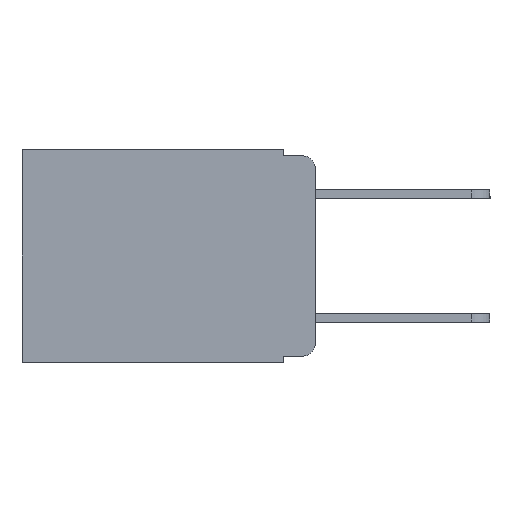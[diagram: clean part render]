
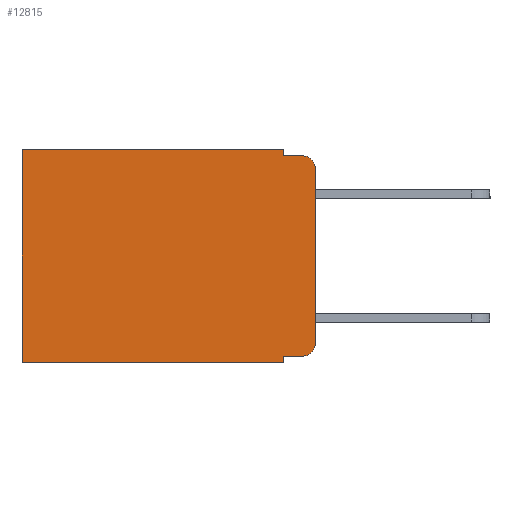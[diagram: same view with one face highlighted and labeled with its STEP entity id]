
A CAD part, left-side view. The second image highlights one B-rep face of the part: STEP entity #12815.
In plain terms, the highlighted planar face has unit normal (-1, 0, 0).
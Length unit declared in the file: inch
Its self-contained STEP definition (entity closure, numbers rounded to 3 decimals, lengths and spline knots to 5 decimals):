
#203 = LINE ( 'NONE', #10145, #24065 ) ;
#232 = AXIS2_PLACEMENT_3D ( 'NONE', #9167, #1278, #14845 ) ;
#376 = FACE_OUTER_BOUND ( 'NONE', #3864, .T. ) ;
#669 = CARTESIAN_POINT ( 'NONE',  ( 0.298, 0.02, -0.01 ) ) ;
#737 = DIRECTION ( 'NONE',  ( 0., 0., -1. ) ) ;
#932 = EDGE_CURVE ( 'NONE', #7446, #4403, #10156, .T. ) ;
#989 = CARTESIAN_POINT ( 'NONE',  ( 0.298, 0.051, -0.333 ) ) ;
#1278 = DIRECTION ( 'NONE',  ( 1., 0., 0. ) ) ;
#1510 = VERTEX_POINT ( 'NONE', #11064 ) ;
#1795 = CARTESIAN_POINT ( 'NONE',  ( 0.298, 0.051, 0. ) ) ;
#1995 = CARTESIAN_POINT ( 'NONE',  ( 0.298, 0.051, -0.01 ) ) ;
#2602 = ORIENTED_EDGE ( 'NONE', *, *, #932, .F. ) ;
#2742 = DIRECTION ( 'NONE',  ( 0., 1., 0. ) ) ;
#3215 = VERTEX_POINT ( 'NONE', #3686 ) ;
#3256 = ORIENTED_EDGE ( 'NONE', *, *, #9403, .T. ) ;
#3280 = ORIENTED_EDGE ( 'NONE', *, *, #9999, .F. ) ;
#3568 = ORIENTED_EDGE ( 'NONE', *, *, #19341, .F. ) ;
#3686 = CARTESIAN_POINT ( 'NONE',  ( 0.298, 0.473, 0. ) ) ;
#3766 = LINE ( 'NONE', #22955, #8368 ) ;
#3864 = EDGE_LOOP ( 'NONE', ( #22841, #7643, #3568, #2602, #13840, #3256, #3280, #7312, #7011, #20078 ) ) ;
#4031 = DIRECTION ( 'NONE',  ( 0., -1., 0. ) ) ;
#4107 = CIRCLE ( 'NONE', #16629, 0.02 ) ;
#4403 = VERTEX_POINT ( 'NONE', #23333 ) ;
#5460 = VERTEX_POINT ( 'NONE', #669 ) ;
#7011 = ORIENTED_EDGE ( 'NONE', *, *, #19006, .T. ) ;
#7312 = ORIENTED_EDGE ( 'NONE', *, *, #20565, .F. ) ;
#7423 = CARTESIAN_POINT ( 'NONE',  ( 0.298, 0.02, -0.333 ) ) ;
#7446 = VERTEX_POINT ( 'NONE', #1795 ) ;
#7643 = ORIENTED_EDGE ( 'NONE', *, *, #13265, .T. ) ;
#8216 = CARTESIAN_POINT ( 'NONE',  ( 0.298, 0.051, 0. ) ) ;
#8368 = VECTOR ( 'NONE', #12138, 39.37008 ) ;
#8554 = VERTEX_POINT ( 'NONE', #20845 ) ;
#8719 = DIRECTION ( 'NONE',  ( -1., 0., 0. ) ) ;
#9006 = LINE ( 'NONE', #1995, #18877 ) ;
#9167 = CARTESIAN_POINT ( 'NONE',  ( 0.298, 0., 0. ) ) ;
#9403 = EDGE_CURVE ( 'NONE', #3215, #8554, #23043, .T. ) ;
#9947 = VERTEX_POINT ( 'NONE', #19228 ) ;
#9999 = EDGE_CURVE ( 'NONE', #1510, #8554, #3766, .T. ) ;
#10145 = CARTESIAN_POINT ( 'NONE',  ( 0.298, 0.051, 0. ) ) ;
#10156 = LINE ( 'NONE', #8216, #22988 ) ;
#10249 = VECTOR ( 'NONE', #2742, 39.37008 ) ;
#10426 = VECTOR ( 'NONE', #10795, 39.37008 ) ;
#10795 = DIRECTION ( 'NONE',  ( 0., 0., -1. ) ) ;
#10827 = CARTESIAN_POINT ( 'NONE',  ( 0.298, 0., -0.313 ) ) ;
#10878 = DIRECTION ( 'NONE',  ( 0., -1., 0. ) ) ;
#10952 = CARTESIAN_POINT ( 'NONE',  ( 0.298, 0.02, -0.313 ) ) ;
#11064 = CARTESIAN_POINT ( 'NONE',  ( 0.298, 0.051, -0.343 ) ) ;
#11135 = PLANE ( 'NONE',  #232 ) ;
#11161 = LINE ( 'NONE', #989, #20289 ) ;
#11203 = EDGE_CURVE ( 'NONE', #11331, #20774, #22689, .T. ) ;
#11331 = VERTEX_POINT ( 'NONE', #7423 ) ;
#11734 = CARTESIAN_POINT ( 'NONE',  ( 0.298, 0., -0.03 ) ) ;
#12138 = DIRECTION ( 'NONE',  ( 0., 1., 0. ) ) ;
#12815 = ADVANCED_FACE ( 'NONE', ( #376 ), #11135, .F. ) ;
#12862 = DIRECTION ( 'NONE',  ( 0., 0., -1. ) ) ;
#13265 = EDGE_CURVE ( 'NONE', #18656, #5460, #4107, .T. ) ;
#13840 = ORIENTED_EDGE ( 'NONE', *, *, #16574, .T. ) ;
#14378 = DIRECTION ( 'NONE',  ( 0., 0., -1. ) ) ;
#14845 = DIRECTION ( 'NONE',  ( 0., 0., -1. ) ) ;
#16159 = CARTESIAN_POINT ( 'NONE',  ( 0.298, 0., 0. ) ) ;
#16574 = EDGE_CURVE ( 'NONE', #7446, #3215, #16935, .T. ) ;
#16629 = AXIS2_PLACEMENT_3D ( 'NONE', #19792, #8719, #21600 ) ;
#16935 = LINE ( 'NONE', #16159, #10249 ) ;
#18085 = CARTESIAN_POINT ( 'NONE',  ( 0.298, 0., 0. ) ) ;
#18656 = VERTEX_POINT ( 'NONE', #11734 ) ;
#18877 = VECTOR ( 'NONE', #4031, 39.37008 ) ;
#19006 = EDGE_CURVE ( 'NONE', #9947, #11331, #11161, .T. ) ;
#19228 = CARTESIAN_POINT ( 'NONE',  ( 0.298, 0.051, -0.333 ) ) ;
#19341 = EDGE_CURVE ( 'NONE', #4403, #5460, #9006, .T. ) ;
#19743 = AXIS2_PLACEMENT_3D ( 'NONE', #10952, #23637, #12862 ) ;
#19792 = CARTESIAN_POINT ( 'NONE',  ( 0.298, 0.02, -0.03 ) ) ;
#20078 = ORIENTED_EDGE ( 'NONE', *, *, #11203, .T. ) ;
#20289 = VECTOR ( 'NONE', #10878, 39.37008 ) ;
#20565 = EDGE_CURVE ( 'NONE', #9947, #1510, #203, .T. ) ;
#20774 = VERTEX_POINT ( 'NONE', #10827 ) ;
#20845 = CARTESIAN_POINT ( 'NONE',  ( 0.298, 0.473, -0.343 ) ) ;
#21132 = DIRECTION ( 'NONE',  ( 0., 0., -1. ) ) ;
#21600 = DIRECTION ( 'NONE',  ( 0., 0., -1. ) ) ;
#22689 = CIRCLE ( 'NONE', #19743, 0.02 ) ;
#22841 = ORIENTED_EDGE ( 'NONE', *, *, #23765, .F. ) ;
#22955 = CARTESIAN_POINT ( 'NONE',  ( 0.298, 0., -0.343 ) ) ;
#22988 = VECTOR ( 'NONE', #737, 39.37008 ) ;
#23043 = LINE ( 'NONE', #23340, #23594 ) ;
#23333 = CARTESIAN_POINT ( 'NONE',  ( 0.298, 0.051, -0.01 ) ) ;
#23340 = CARTESIAN_POINT ( 'NONE',  ( 0.298, 0.473, 0. ) ) ;
#23594 = VECTOR ( 'NONE', #14378, 39.37008 ) ;
#23637 = DIRECTION ( 'NONE',  ( -1., 0., 0. ) ) ;
#23765 = EDGE_CURVE ( 'NONE', #18656, #20774, #24308, .T. ) ;
#24065 = VECTOR ( 'NONE', #21132, 39.37008 ) ;
#24308 = LINE ( 'NONE', #18085, #10426 ) ;
